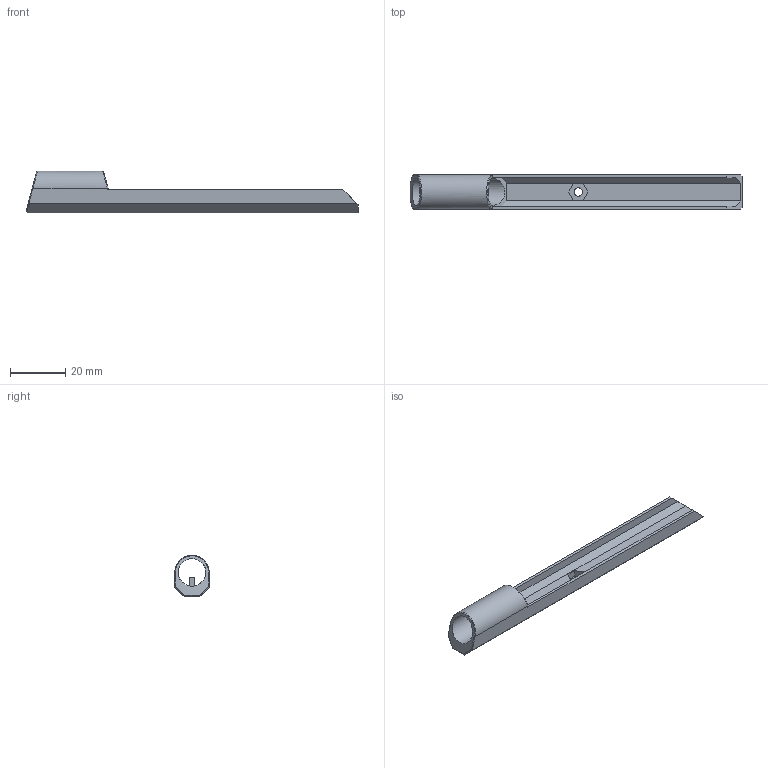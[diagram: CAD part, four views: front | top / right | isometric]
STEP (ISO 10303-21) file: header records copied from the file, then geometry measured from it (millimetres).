
FILE_DESCRIPTION(/* description */ (''),/* implementation_level */ '2;1');
FILE_NAME(/* name */ 'Carry Handle Sight.step',/* time_stamp */ '2022-06-02T14:07:51-06:00',/* author */ (''),/* organization */ (''),/* preprocessor_version */ 'ST-DEVELOPER v19',/* originating_system */ 'Autodesk Translation Framework v11.7.0.108',/* authorisation */ '');
FILE_SCHEMA (('AUTOMOTIVE_DESIGN { 1 0 10303 214 3 1 1 }'));
Length unit declared in the file: millimetre
Products named in the file (1): M16K Sight
Bounding box: 120.37 x 12.5 x 15.1 mm (x, y, z)
Volume: 6356.3 mm3; surface area: 6406 mm2
Topology: 1 solids, 1 shells, 45 faces, 122 edges, 80 vertices
Faces by surface type: plane 36, bspline 6, cylinder 3
Full cylindrical faces by diameter (mm): 3 x1, 10 x1
Entity records: 1590 total; most frequent: CARTESIAN_POINT 440, ORIENTED_EDGE 244, DIRECTION 198, EDGE_CURVE 122, LINE 102, VECTOR 102, VERTEX_POINT 80, EDGE_LOOP 50
